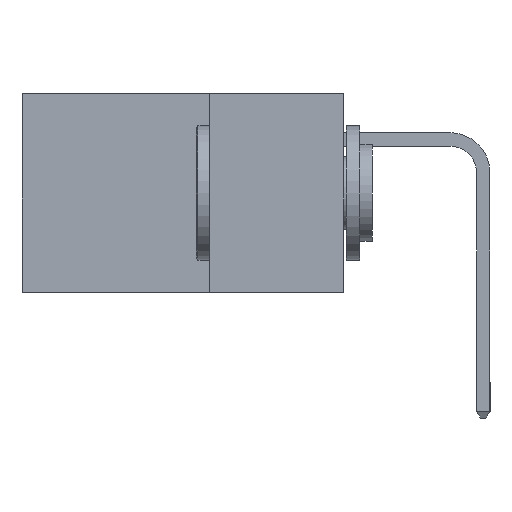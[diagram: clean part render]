
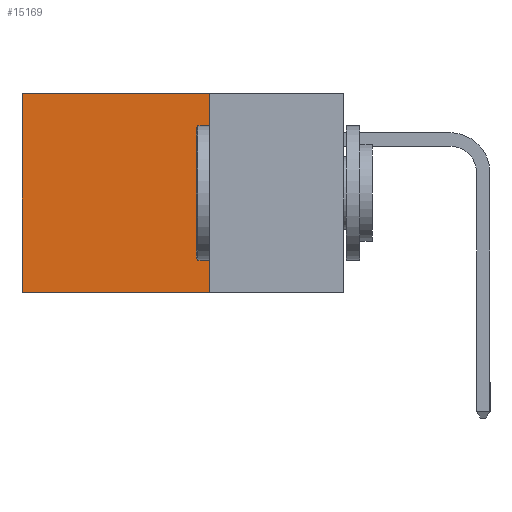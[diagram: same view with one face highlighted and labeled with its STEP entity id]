
A CAD part, left-side view. The second image highlights one B-rep face of the part: STEP entity #15169.
In plain terms, the highlighted planar face has unit normal (-1, 0, 0).
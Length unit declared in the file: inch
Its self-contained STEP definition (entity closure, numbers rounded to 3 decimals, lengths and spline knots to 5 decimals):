
#34 = EDGE_CURVE ( 'NONE', #4326, #6293, #6704, .T. ) ;
#538 = VECTOR ( 'NONE', #5685, 39.37008 ) ;
#2122 = EDGE_LOOP ( 'NONE', ( #11547, #2150, #8759, #2633 ) ) ;
#2150 = ORIENTED_EDGE ( 'NONE', *, *, #2981, .F. ) ;
#2633 = ORIENTED_EDGE ( 'NONE', *, *, #34, .T. ) ;
#2981 = EDGE_CURVE ( 'NONE', #5658, #9396, #9516, .T. ) ;
#3662 = CARTESIAN_POINT ( 'NONE',  ( 0.298, 0.6, 0. ) ) ;
#4326 = VERTEX_POINT ( 'NONE', #9377 ) ;
#5363 = CARTESIAN_POINT ( 'NONE',  ( 0.298, 0.25, 0. ) ) ;
#5407 = LINE ( 'NONE', #3662, #8265 ) ;
#5414 = DIRECTION ( 'NONE',  ( 1., 0., 0. ) ) ;
#5658 = VERTEX_POINT ( 'NONE', #15864 ) ;
#5685 = DIRECTION ( 'NONE',  ( 0., 1., 0. ) ) ;
#6293 = VERTEX_POINT ( 'NONE', #15795 ) ;
#6704 = LINE ( 'NONE', #15001, #538 ) ;
#6930 = EDGE_CURVE ( 'NONE', #4326, #5658, #8681, .T. ) ;
#6986 = DIRECTION ( 'NONE',  ( 0., 0., -1. ) ) ;
#7308 = DIRECTION ( 'NONE',  ( 0., 0., -1. ) ) ;
#7421 = VECTOR ( 'NONE', #14131, 39.37008 ) ;
#8159 = FACE_OUTER_BOUND ( 'NONE', #2122, .T. ) ;
#8265 = VECTOR ( 'NONE', #7308, 39.37008 ) ;
#8681 = LINE ( 'NONE', #12970, #14896 ) ;
#8759 = ORIENTED_EDGE ( 'NONE', *, *, #6930, .F. ) ;
#9377 = CARTESIAN_POINT ( 'NONE',  ( 0.298, 0.25, 0. ) ) ;
#9396 = VERTEX_POINT ( 'NONE', #15339 ) ;
#9481 = EDGE_CURVE ( 'NONE', #6293, #9396, #5407, .T. ) ;
#9516 = LINE ( 'NONE', #14005, #7421 ) ;
#10253 = PLANE ( 'NONE',  #12693 ) ;
#11547 = ORIENTED_EDGE ( 'NONE', *, *, #9481, .T. ) ;
#12693 = AXIS2_PLACEMENT_3D ( 'NONE', #5363, #5414, #13778 ) ;
#12970 = CARTESIAN_POINT ( 'NONE',  ( 0.298, 0.25, 0. ) ) ;
#13778 = DIRECTION ( 'NONE',  ( 0., 0., -1. ) ) ;
#14005 = CARTESIAN_POINT ( 'NONE',  ( 0.298, 0.25, -0.37 ) ) ;
#14131 = DIRECTION ( 'NONE',  ( 0., 1., 0. ) ) ;
#14896 = VECTOR ( 'NONE', #6986, 39.37008 ) ;
#15001 = CARTESIAN_POINT ( 'NONE',  ( 0.298, 0.25, 0. ) ) ;
#15169 = ADVANCED_FACE ( 'NONE', ( #8159 ), #10253, .F. ) ;
#15339 = CARTESIAN_POINT ( 'NONE',  ( 0.298, 0.6, -0.37 ) ) ;
#15795 = CARTESIAN_POINT ( 'NONE',  ( 0.298, 0.6, 0. ) ) ;
#15864 = CARTESIAN_POINT ( 'NONE',  ( 0.298, 0.25, -0.37 ) ) ;
